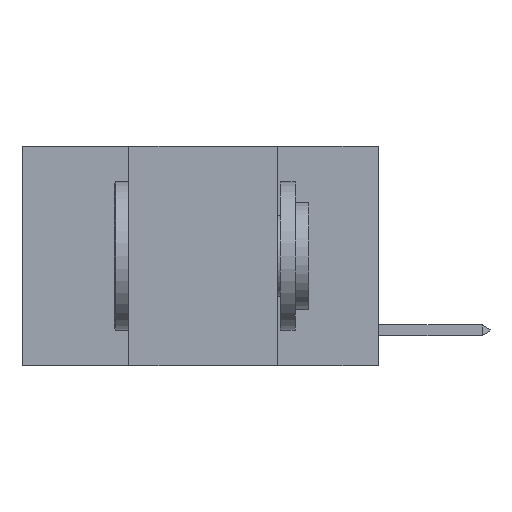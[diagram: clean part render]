
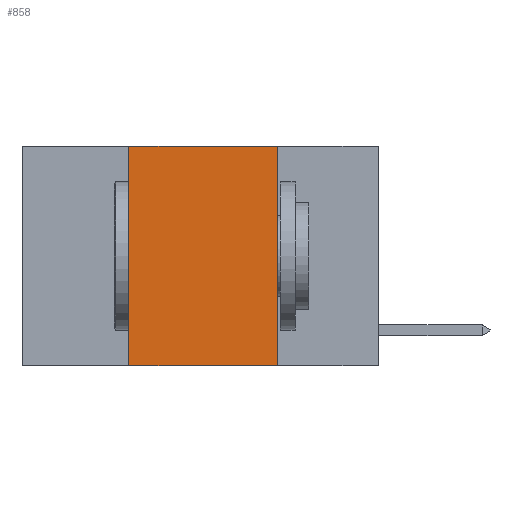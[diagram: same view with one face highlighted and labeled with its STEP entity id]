
A CAD part, left-side view. The second image highlights one B-rep face of the part: STEP entity #858.
In plain terms, the highlighted planar face has unit normal (-1, 0, 0).
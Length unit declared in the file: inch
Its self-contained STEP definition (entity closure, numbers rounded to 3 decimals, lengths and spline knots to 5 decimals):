
#858 = ADVANCED_FACE ( 'NONE', ( #5921 ), #22242, .F. ) ;
#4251 = CARTESIAN_POINT ( 'NONE',  ( 0., 0.17, -0.37 ) ) ;
#4923 = CARTESIAN_POINT ( 'NONE',  ( 0., 0.42, 0. ) ) ;
#5015 = EDGE_CURVE ( 'NONE', #21756, #6980, #27949, .T. ) ;
#5767 = DIRECTION ( 'NONE',  ( 1., 0., 0. ) ) ;
#5921 = FACE_OUTER_BOUND ( 'NONE', #13040, .T. ) ;
#6264 = CARTESIAN_POINT ( 'NONE',  ( 0., 0.6, 0. ) ) ;
#6980 = VERTEX_POINT ( 'NONE', #10981 ) ;
#7864 = DIRECTION ( 'NONE',  ( 0., 0., -1. ) ) ;
#8457 = VECTOR ( 'NONE', #7864, 39.37008 ) ;
#9156 = AXIS2_PLACEMENT_3D ( 'NONE', #17493, #5767, #10208 ) ;
#9446 = VECTOR ( 'NONE', #26460, 39.37008 ) ;
#10143 = CARTESIAN_POINT ( 'NONE',  ( 0., 0.42, -0.37 ) ) ;
#10208 = DIRECTION ( 'NONE',  ( 0., 0., -1. ) ) ;
#10981 = CARTESIAN_POINT ( 'NONE',  ( 0., 0.17, 0. ) ) ;
#11200 = EDGE_CURVE ( 'NONE', #25615, #21756, #24393, .T. ) ;
#11352 = VECTOR ( 'NONE', #20829, 39.37008 ) ;
#11685 = EDGE_CURVE ( 'NONE', #6980, #12826, #12613, .T. ) ;
#12613 = LINE ( 'NONE', #30007, #8457 ) ;
#12764 = ORIENTED_EDGE ( 'NONE', *, *, #11200, .F. ) ;
#12826 = VERTEX_POINT ( 'NONE', #4251 ) ;
#13040 = EDGE_LOOP ( 'NONE', ( #20027, #21022, #12764, #18936 ) ) ;
#16375 = EDGE_CURVE ( 'NONE', #25615, #12826, #27979, .T. ) ;
#16789 = CARTESIAN_POINT ( 'NONE',  ( 0., 0.42, 0. ) ) ;
#17493 = CARTESIAN_POINT ( 'NONE',  ( 0., 0.6, 0. ) ) ;
#18936 = ORIENTED_EDGE ( 'NONE', *, *, #16375, .T. ) ;
#20027 = ORIENTED_EDGE ( 'NONE', *, *, #11685, .F. ) ;
#20829 = DIRECTION ( 'NONE',  ( 0., -1., 0. ) ) ;
#20865 = CARTESIAN_POINT ( 'NONE',  ( 0., 0.6, -0.37 ) ) ;
#21022 = ORIENTED_EDGE ( 'NONE', *, *, #5015, .F. ) ;
#21756 = VERTEX_POINT ( 'NONE', #4923 ) ;
#22242 = PLANE ( 'NONE',  #9156 ) ;
#23265 = VECTOR ( 'NONE', #30506, 39.37008 ) ;
#24393 = LINE ( 'NONE', #16789, #9446 ) ;
#25615 = VERTEX_POINT ( 'NONE', #10143 ) ;
#26460 = DIRECTION ( 'NONE',  ( 0., 0., 1. ) ) ;
#27949 = LINE ( 'NONE', #6264, #11352 ) ;
#27979 = LINE ( 'NONE', #20865, #23265 ) ;
#30007 = CARTESIAN_POINT ( 'NONE',  ( 0., 0.17, 0. ) ) ;
#30506 = DIRECTION ( 'NONE',  ( 0., -1., 0. ) ) ;
